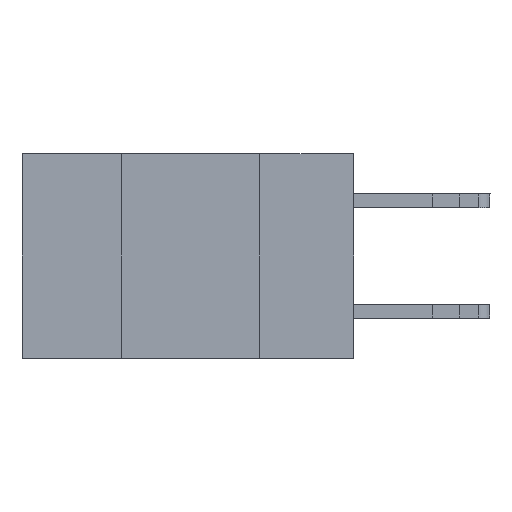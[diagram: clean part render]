
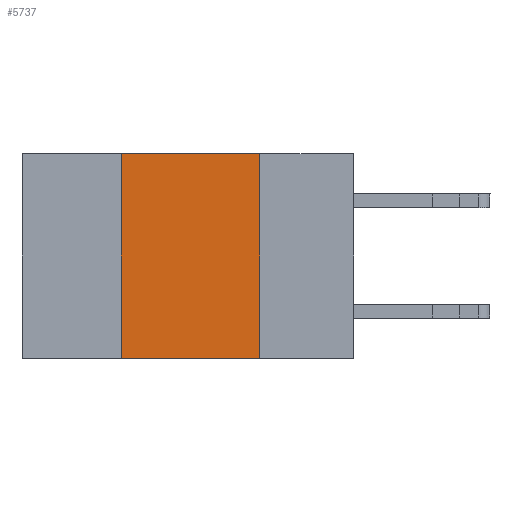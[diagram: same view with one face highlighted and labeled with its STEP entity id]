
A CAD part, left-side view. The second image highlights one B-rep face of the part: STEP entity #5737.
In plain terms, the highlighted planar face has unit normal (-1, 0, 0).
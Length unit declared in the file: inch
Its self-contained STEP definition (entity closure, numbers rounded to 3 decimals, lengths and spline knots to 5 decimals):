
#128 = EDGE_CURVE ( 'NONE', #5361, #17885, #2673, .T. ) ;
#584 = EDGE_CURVE ( 'NONE', #12451, #15335, #12709, .T. ) ;
#668 = DIRECTION ( 'NONE',  ( 0., 0., 1. ) ) ;
#1587 = CARTESIAN_POINT ( 'NONE',  ( 0., 0.6, 0. ) ) ;
#1921 = CARTESIAN_POINT ( 'NONE',  ( 0., 0.17, 0. ) ) ;
#2673 = LINE ( 'NONE', #7383, #16600 ) ;
#2815 = CARTESIAN_POINT ( 'NONE',  ( 0., 0.42, 0. ) ) ;
#3009 = DIRECTION ( 'NONE',  ( 0., -1., 0. ) ) ;
#5013 = DIRECTION ( 'NONE',  ( 0., -1., 0. ) ) ;
#5361 = VERTEX_POINT ( 'NONE', #8514 ) ;
#5737 = ADVANCED_FACE ( 'NONE', ( #17686 ), #7438, .F. ) ;
#6135 = VECTOR ( 'NONE', #3009, 39.37008 ) ;
#7101 = VECTOR ( 'NONE', #5013, 39.37008 ) ;
#7383 = CARTESIAN_POINT ( 'NONE',  ( 0., 0.42, 0. ) ) ;
#7438 = PLANE ( 'NONE',  #19581 ) ;
#7880 = DIRECTION ( 'NONE',  ( 1., 0., 0. ) ) ;
#8514 = CARTESIAN_POINT ( 'NONE',  ( 0., 0.42, -0.37 ) ) ;
#8727 = EDGE_LOOP ( 'NONE', ( #10564, #18030, #15058, #10235 ) ) ;
#9606 = CARTESIAN_POINT ( 'NONE',  ( 0., 0.6, 0. ) ) ;
#10235 = ORIENTED_EDGE ( 'NONE', *, *, #13577, .T. ) ;
#10564 = ORIENTED_EDGE ( 'NONE', *, *, #584, .F. ) ;
#11035 = CARTESIAN_POINT ( 'NONE',  ( 0., 0.17, 0. ) ) ;
#12451 = VERTEX_POINT ( 'NONE', #1921 ) ;
#12709 = LINE ( 'NONE', #11035, #17382 ) ;
#12925 = DIRECTION ( 'NONE',  ( 0., 0., -1. ) ) ;
#13577 = EDGE_CURVE ( 'NONE', #5361, #15335, #17490, .T. ) ;
#14464 = EDGE_CURVE ( 'NONE', #17885, #12451, #19979, .T. ) ;
#15058 = ORIENTED_EDGE ( 'NONE', *, *, #128, .F. ) ;
#15335 = VERTEX_POINT ( 'NONE', #20316 ) ;
#16600 = VECTOR ( 'NONE', #668, 39.37008 ) ;
#17382 = VECTOR ( 'NONE', #19478, 39.37008 ) ;
#17490 = LINE ( 'NONE', #17945, #6135 ) ;
#17686 = FACE_OUTER_BOUND ( 'NONE', #8727, .T. ) ;
#17885 = VERTEX_POINT ( 'NONE', #2815 ) ;
#17945 = CARTESIAN_POINT ( 'NONE',  ( 0., 0.6, -0.37 ) ) ;
#18030 = ORIENTED_EDGE ( 'NONE', *, *, #14464, .F. ) ;
#19478 = DIRECTION ( 'NONE',  ( 0., 0., -1. ) ) ;
#19581 = AXIS2_PLACEMENT_3D ( 'NONE', #9606, #7880, #12925 ) ;
#19979 = LINE ( 'NONE', #1587, #7101 ) ;
#20316 = CARTESIAN_POINT ( 'NONE',  ( 0., 0.17, -0.37 ) ) ;
